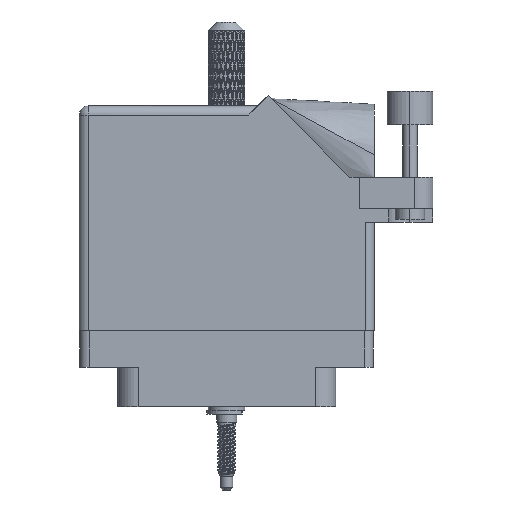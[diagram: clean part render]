
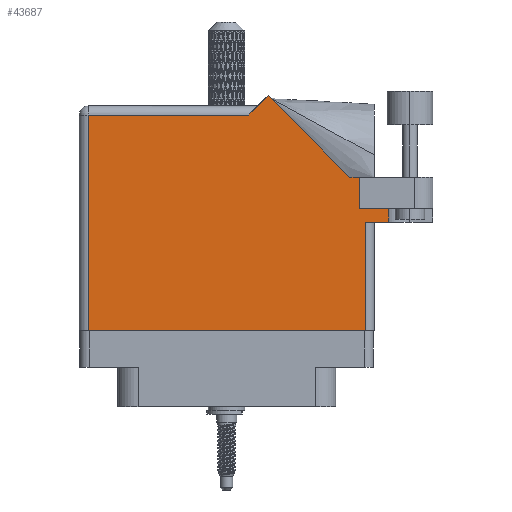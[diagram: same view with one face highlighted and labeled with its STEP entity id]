
A CAD part, front view. The second image highlights one B-rep face of the part: STEP entity #43687.
In plain terms, the highlighted face is planar.
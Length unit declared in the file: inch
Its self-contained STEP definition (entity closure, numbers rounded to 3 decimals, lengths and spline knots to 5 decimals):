
#1485 = VECTOR ( 'NONE', #4301, 39.37008 ) ;
#4301 = DIRECTION ( 'NONE',  ( 0., 1., 0. ) ) ;
#5765 = CARTESIAN_POINT ( 'NONE',  ( 0.943, 0.637, 0.455 ) ) ;
#6345 = CARTESIAN_POINT ( 'NONE',  ( 0.905, 0.731, 0.455 ) ) ;
#7766 = AXIS2_PLACEMENT_3D ( 'NONE', #98066, #48128, #80902 ) ;
#7974 = LINE ( 'NONE', #38649, #105304 ) ;
#9068 = EDGE_CURVE ( 'NONE', #52967, #35229, #76839, .T. ) ;
#10745 = LINE ( 'NONE', #17753, #96346 ) ;
#11175 = DIRECTION ( 'NONE',  ( 1., 0., 0. ) ) ;
#11373 = DIRECTION ( 'NONE',  ( -1., 0., 0. ) ) ;
#12242 = LINE ( 'NONE', #43982, #54872 ) ;
#13628 = VECTOR ( 'NONE', #14571, 39.37008 ) ;
#13709 = EDGE_CURVE ( 'NONE', #60750, #17905, #12242, .T. ) ;
#14261 = CARTESIAN_POINT ( 'NONE',  ( -0.943, -0.1, 0.455 ) ) ;
#14571 = DIRECTION ( 'NONE',  ( 1., 0., 0. ) ) ;
#16408 = PLANE ( 'NONE',  #7766 ) ;
#16582 = LINE ( 'NONE', #48836, #88993 ) ;
#17682 = LINE ( 'NONE', #51495, #83951 ) ;
#17753 = CARTESIAN_POINT ( 'NONE',  ( 0.212, 1.43, 0.455 ) ) ;
#17905 = VERTEX_POINT ( 'NONE', #47635 ) ;
#19262 = EDGE_CURVE ( 'NONE', #35229, #34462, #94490, .T. ) ;
#19306 = VERTEX_POINT ( 'NONE', #31613 ) ;
#20665 = ORIENTED_EDGE ( 'NONE', *, *, #53364, .T. ) ;
#21510 = VERTEX_POINT ( 'NONE', #57307 ) ;
#27376 = ORIENTED_EDGE ( 'NONE', *, *, #105816, .F. ) ;
#27377 = DIRECTION ( 'NONE',  ( -0.707, 0.707, 0. ) ) ;
#27787 = VECTOR ( 'NONE', #88562, 39.37008 ) ;
#30592 = DIRECTION ( 'NONE',  ( -1., 0., 0. ) ) ;
#31539 = EDGE_LOOP ( 'NONE', ( #54655, #81682, #53463, #27376, #71359, #80720, #39328, #20665, #37479, #82189, #95423 ) ) ;
#31613 = CARTESIAN_POINT ( 'NONE',  ( 0.905, 0.944, 0.455 ) ) ;
#33065 = FACE_OUTER_BOUND ( 'NONE', #31539, .T. ) ;
#34462 = VERTEX_POINT ( 'NONE', #99712 ) ;
#35229 = VERTEX_POINT ( 'NONE', #5765 ) ;
#36071 = VERTEX_POINT ( 'NONE', #14261 ) ;
#36535 = CARTESIAN_POINT ( 'NONE',  ( 0.943, 0.637, 0.455 ) ) ;
#37479 = ORIENTED_EDGE ( 'NONE', *, *, #87030, .T. ) ;
#38649 = CARTESIAN_POINT ( 'NONE',  ( 1.405, 0.944, 0.455 ) ) ;
#39328 = ORIENTED_EDGE ( 'NONE', *, *, #96146, .T. ) ;
#39704 = CARTESIAN_POINT ( 'NONE',  ( 0.28271, 1.50071, 0.455 ) ) ;
#43687 = ADVANCED_FACE ( 'NONE', ( #33065 ), #16408, .F. ) ;
#43982 = CARTESIAN_POINT ( 'NONE',  ( 0.905, 0.731, 0.455 ) ) ;
#45149 = CARTESIAN_POINT ( 'NONE',  ( 0.905, 0.731, 0.455 ) ) ;
#46931 = EDGE_CURVE ( 'NONE', #36071, #52967, #80638, .T. ) ;
#47635 = CARTESIAN_POINT ( 'NONE',  ( 1.1065, 0.731, 0.455 ) ) ;
#48128 = DIRECTION ( 'NONE',  ( 0., 0., -1. ) ) ;
#48836 = CARTESIAN_POINT ( 'NONE',  ( -0.943, -0.1, 0.455 ) ) ;
#49887 = DIRECTION ( 'NONE',  ( 0., -1., 0. ) ) ;
#50646 = LINE ( 'NONE', #60248, #79479 ) ;
#51495 = CARTESIAN_POINT ( 'NONE',  ( 1.1065, 1.06177, 0.455 ) ) ;
#52967 = VERTEX_POINT ( 'NONE', #74836 ) ;
#53364 = EDGE_CURVE ( 'NONE', #78478, #67446, #68200, .T. ) ;
#53463 = ORIENTED_EDGE ( 'NONE', *, *, #19262, .T. ) ;
#54655 = ORIENTED_EDGE ( 'NONE', *, *, #46931, .T. ) ;
#54872 = VECTOR ( 'NONE', #11175, 39.37008 ) ;
#57307 = CARTESIAN_POINT ( 'NONE',  ( 0.15, 1.368, 0.455 ) ) ;
#60248 = CARTESIAN_POINT ( 'NONE',  ( -1.005, 1.368, 0.455 ) ) ;
#60306 = VERTEX_POINT ( 'NONE', #88279 ) ;
#60750 = VERTEX_POINT ( 'NONE', #6345 ) ;
#67157 = DIRECTION ( 'NONE',  ( -0.707, -0.707, 0. ) ) ;
#67446 = VERTEX_POINT ( 'NONE', #39704 ) ;
#68200 = LINE ( 'NONE', #69297, #93053 ) ;
#69297 = CARTESIAN_POINT ( 'NONE',  ( 0.83942, 0.944, 0.455 ) ) ;
#70565 = CARTESIAN_POINT ( 'NONE',  ( 0.83942, 0.944, 0.455 ) ) ;
#71359 = ORIENTED_EDGE ( 'NONE', *, *, #13709, .F. ) ;
#72451 = CARTESIAN_POINT ( 'NONE',  ( 1.005, 0.637, 0.455 ) ) ;
#74836 = CARTESIAN_POINT ( 'NONE',  ( 0.943, -0.1, 0.455 ) ) ;
#76299 = DIRECTION ( 'NONE',  ( 0., 1., 0. ) ) ;
#76839 = LINE ( 'NONE', #36535, #83713 ) ;
#78478 = VERTEX_POINT ( 'NONE', #70565 ) ;
#79479 = VECTOR ( 'NONE', #11373, 39.37008 ) ;
#80638 = LINE ( 'NONE', #105351, #13628 ) ;
#80720 = ORIENTED_EDGE ( 'NONE', *, *, #81305, .T. ) ;
#80902 = DIRECTION ( 'NONE',  ( -1., 0., 0. ) ) ;
#81305 = EDGE_CURVE ( 'NONE', #60750, #19306, #93480, .T. ) ;
#81513 = EDGE_CURVE ( 'NONE', #60306, #36071, #16582, .T. ) ;
#81682 = ORIENTED_EDGE ( 'NONE', *, *, #9068, .T. ) ;
#82189 = ORIENTED_EDGE ( 'NONE', *, *, #95557, .T. ) ;
#83713 = VECTOR ( 'NONE', #76299, 39.37008 ) ;
#83951 = VECTOR ( 'NONE', #99341, 39.37008 ) ;
#87030 = EDGE_CURVE ( 'NONE', #67446, #21510, #10745, .T. ) ;
#88279 = CARTESIAN_POINT ( 'NONE',  ( -0.943, 1.368, 0.455 ) ) ;
#88562 = DIRECTION ( 'NONE',  ( 1., 0., 0. ) ) ;
#88993 = VECTOR ( 'NONE', #49887, 39.37008 ) ;
#93053 = VECTOR ( 'NONE', #27377, 39.37008 ) ;
#93480 = LINE ( 'NONE', #45149, #1485 ) ;
#94490 = LINE ( 'NONE', #72451, #27787 ) ;
#95423 = ORIENTED_EDGE ( 'NONE', *, *, #81513, .T. ) ;
#95557 = EDGE_CURVE ( 'NONE', #21510, #60306, #50646, .T. ) ;
#96146 = EDGE_CURVE ( 'NONE', #19306, #78478, #7974, .T. ) ;
#96346 = VECTOR ( 'NONE', #67157, 39.37008 ) ;
#98066 = CARTESIAN_POINT ( 'NONE',  ( -1.005, 1.43, 0.455 ) ) ;
#99341 = DIRECTION ( 'NONE',  ( 0., -1., 0. ) ) ;
#99712 = CARTESIAN_POINT ( 'NONE',  ( 1.1065, 0.637, 0.455 ) ) ;
#105304 = VECTOR ( 'NONE', #30592, 39.37008 ) ;
#105351 = CARTESIAN_POINT ( 'NONE',  ( -1.005, -0.1, 0.455 ) ) ;
#105816 = EDGE_CURVE ( 'NONE', #17905, #34462, #17682, .T. ) ;
